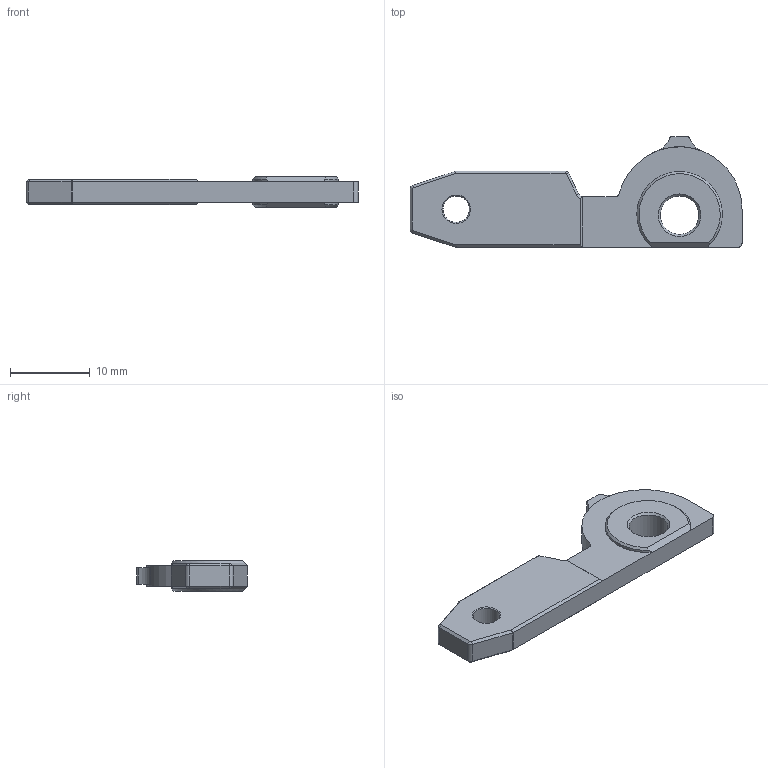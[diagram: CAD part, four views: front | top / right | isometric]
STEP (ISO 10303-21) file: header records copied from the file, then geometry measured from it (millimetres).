
FILE_DESCRIPTION(/* description */ (''),/* implementation_level */ '2;1');
FILE_NAME(/* name */ 'SSL v6.step',/* time_stamp */ '2021-04-20T06:57:46-05:00',/* author */ (''),/* organization */ (''),/* preprocessor_version */ 'ST-DEVELOPER v18.1',/* originating_system */ 'Autodesk Translation Framework v10.6.0.1341',/* authorisation */ '');
FILE_SCHEMA (('AUTOMOTIVE_DESIGN { 1 0 10303 214 3 1 1 }'));
Length unit declared in the file: inch
Products named in the file (1): SSL
Bounding box: 41.53 x 13.84 x 3.76 mm (x, y, z)
Volume: 1119.9 mm3; surface area: 1125.8 mm2
Topology: 1 solids, 1 shells, 68 faces, 163 edges, 98 vertices
Faces by surface type: plane 33, cone 18, cylinder 17
Full cylindrical faces by diameter (mm): 3.302 x1, 4.826 x1
Entity records: 1984 total; most frequent: DIRECTION 351, CARTESIAN_POINT 346, ORIENTED_EDGE 326, EDGE_CURVE 163, AXIS2_PLACEMENT_3D 127, VERTEX_POINT 98, LINE 97, VECTOR 97
